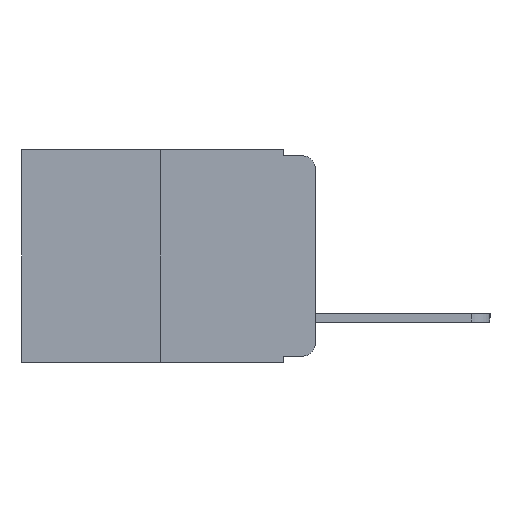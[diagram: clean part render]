
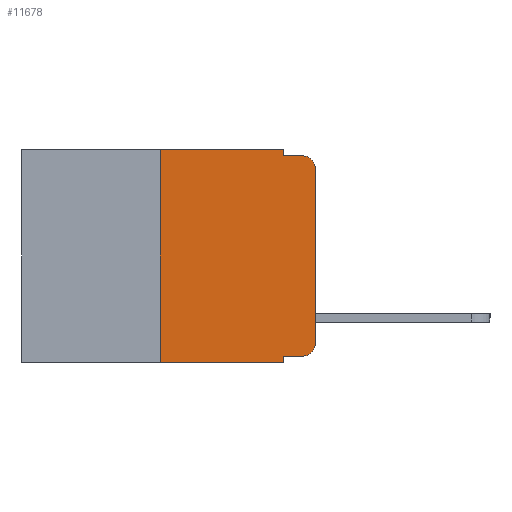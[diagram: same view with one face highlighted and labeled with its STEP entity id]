
A CAD part, left-side view. The second image highlights one B-rep face of the part: STEP entity #11678.
In plain terms, the highlighted planar face has unit normal (-1, 0, 0).
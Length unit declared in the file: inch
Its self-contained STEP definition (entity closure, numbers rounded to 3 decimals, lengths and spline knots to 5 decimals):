
#26 = DIRECTION ( 'NONE',  ( 0., 0., -1. ) ) ;
#235 = ORIENTED_EDGE ( 'NONE', *, *, #14820, .F. ) ;
#338 = DIRECTION ( 'NONE',  ( 1., 0., 0. ) ) ;
#507 = CARTESIAN_POINT ( 'NONE',  ( 0., 0.02, -0.01 ) ) ;
#1001 = DIRECTION ( 'NONE',  ( 0., -1., 0. ) ) ;
#1070 = ORIENTED_EDGE ( 'NONE', *, *, #17965, .F. ) ;
#1415 = DIRECTION ( 'NONE',  ( 0., 0., -1. ) ) ;
#1560 = CARTESIAN_POINT ( 'NONE',  ( 0., 0., 0. ) ) ;
#1815 = CARTESIAN_POINT ( 'NONE',  ( 0., 0.25, -0.343 ) ) ;
#1940 = VERTEX_POINT ( 'NONE', #16878 ) ;
#2002 = PLANE ( 'NONE',  #14987 ) ;
#2041 = VECTOR ( 'NONE', #6393, 39.37008 ) ;
#2504 = EDGE_CURVE ( 'NONE', #9004, #8777, #14650, .T. ) ;
#2697 = VERTEX_POINT ( 'NONE', #507 ) ;
#2746 = CARTESIAN_POINT ( 'NONE',  ( 0., 0.051, -0.333 ) ) ;
#2930 = ORIENTED_EDGE ( 'NONE', *, *, #12748, .T. ) ;
#2942 = FACE_OUTER_BOUND ( 'NONE', #18625, .T. ) ;
#4654 = VERTEX_POINT ( 'NONE', #9263 ) ;
#5141 = DIRECTION ( 'NONE',  ( 0., 0., 1. ) ) ;
#5259 = CARTESIAN_POINT ( 'NONE',  ( 0., 0.051, -0.01 ) ) ;
#5276 = VERTEX_POINT ( 'NONE', #15766 ) ;
#5725 = ORIENTED_EDGE ( 'NONE', *, *, #13641, .T. ) ;
#5962 = LINE ( 'NONE', #2746, #14528 ) ;
#5964 = LINE ( 'NONE', #11373, #14036 ) ;
#6369 = VECTOR ( 'NONE', #18024, 39.37008 ) ;
#6393 = DIRECTION ( 'NONE',  ( 0., 0., -1. ) ) ;
#6933 = CARTESIAN_POINT ( 'NONE',  ( 0., 0.473, 0. ) ) ;
#6975 = DIRECTION ( 'NONE',  ( 0., -1., 0. ) ) ;
#7936 = DIRECTION ( 'NONE',  ( 0., 0., -1. ) ) ;
#8777 = VERTEX_POINT ( 'NONE', #18699 ) ;
#8801 = CARTESIAN_POINT ( 'NONE',  ( 0., 0.051, -0.343 ) ) ;
#8851 = LINE ( 'NONE', #9237, #20805 ) ;
#9004 = VERTEX_POINT ( 'NONE', #17749 ) ;
#9237 = CARTESIAN_POINT ( 'NONE',  ( 0., 0.473, -0.343 ) ) ;
#9263 = CARTESIAN_POINT ( 'NONE',  ( 0., 0.051, -0.01 ) ) ;
#9523 = EDGE_CURVE ( 'NONE', #19681, #9004, #12698, .T. ) ;
#9581 = CARTESIAN_POINT ( 'NONE',  ( 0., 0.051, 0. ) ) ;
#9985 = DIRECTION ( 'NONE',  ( -1., 0., 0. ) ) ;
#10102 = VECTOR ( 'NONE', #7936, 39.37008 ) ;
#10228 = LINE ( 'NONE', #5259, #6369 ) ;
#10261 = LINE ( 'NONE', #14430, #2041 ) ;
#10433 = VECTOR ( 'NONE', #5141, 39.37008 ) ;
#10814 = CARTESIAN_POINT ( 'NONE',  ( 0., 0.051, 0. ) ) ;
#11120 = AXIS2_PLACEMENT_3D ( 'NONE', #20524, #11228, #1415 ) ;
#11228 = DIRECTION ( 'NONE',  ( -1., 0., 0. ) ) ;
#11373 = CARTESIAN_POINT ( 'NONE',  ( 0., 0.25, 0. ) ) ;
#11595 = ORIENTED_EDGE ( 'NONE', *, *, #9523, .T. ) ;
#11678 = ADVANCED_FACE ( 'NONE', ( #2942 ), #2002, .F. ) ;
#11856 = DIRECTION ( 'NONE',  ( 0., 0., -1. ) ) ;
#12392 = VECTOR ( 'NONE', #6975, 39.37008 ) ;
#12394 = VERTEX_POINT ( 'NONE', #1815 ) ;
#12698 = CIRCLE ( 'NONE', #11120, 0.02 ) ;
#12748 = EDGE_CURVE ( 'NONE', #5276, #19681, #5962, .T. ) ;
#12841 = ORIENTED_EDGE ( 'NONE', *, *, #13441, .F. ) ;
#12970 = DIRECTION ( 'NONE',  ( 0., 0., 1. ) ) ;
#13441 = EDGE_CURVE ( 'NONE', #1940, #14596, #16560, .T. ) ;
#13491 = VERTEX_POINT ( 'NONE', #8801 ) ;
#13641 = EDGE_CURVE ( 'NONE', #12394, #13491, #8851, .T. ) ;
#13760 = EDGE_CURVE ( 'NONE', #5276, #13491, #15315, .T. ) ;
#14011 = AXIS2_PLACEMENT_3D ( 'NONE', #19357, #9985, #26 ) ;
#14036 = VECTOR ( 'NONE', #12970, 39.37008 ) ;
#14062 = DIRECTION ( 'NONE',  ( 0., -1., 0. ) ) ;
#14430 = CARTESIAN_POINT ( 'NONE',  ( 0., 0.051, 0. ) ) ;
#14514 = ORIENTED_EDGE ( 'NONE', *, *, #2504, .T. ) ;
#14528 = VECTOR ( 'NONE', #14062, 39.37008 ) ;
#14534 = ORIENTED_EDGE ( 'NONE', *, *, #16960, .F. ) ;
#14596 = VERTEX_POINT ( 'NONE', #10814 ) ;
#14650 = LINE ( 'NONE', #1560, #10433 ) ;
#14820 = EDGE_CURVE ( 'NONE', #12394, #1940, #5964, .T. ) ;
#14862 = CIRCLE ( 'NONE', #14011, 0.02 ) ;
#14987 = AXIS2_PLACEMENT_3D ( 'NONE', #6933, #338, #11856 ) ;
#15315 = LINE ( 'NONE', #9581, #10102 ) ;
#15766 = CARTESIAN_POINT ( 'NONE',  ( 0., 0.051, -0.333 ) ) ;
#16017 = ORIENTED_EDGE ( 'NONE', *, *, #19982, .T. ) ;
#16560 = LINE ( 'NONE', #18120, #12392 ) ;
#16878 = CARTESIAN_POINT ( 'NONE',  ( 0., 0.25, 0. ) ) ;
#16960 = EDGE_CURVE ( 'NONE', #14596, #4654, #10261, .T. ) ;
#17749 = CARTESIAN_POINT ( 'NONE',  ( 0., 0., -0.313 ) ) ;
#17965 = EDGE_CURVE ( 'NONE', #4654, #2697, #10228, .T. ) ;
#18024 = DIRECTION ( 'NONE',  ( 0., -1., 0. ) ) ;
#18120 = CARTESIAN_POINT ( 'NONE',  ( 0., 0.473, 0. ) ) ;
#18625 = EDGE_LOOP ( 'NONE', ( #14514, #16017, #1070, #14534, #12841, #235, #5725, #18938, #2930, #11595 ) ) ;
#18699 = CARTESIAN_POINT ( 'NONE',  ( 0., 0., -0.03 ) ) ;
#18938 = ORIENTED_EDGE ( 'NONE', *, *, #13760, .F. ) ;
#19357 = CARTESIAN_POINT ( 'NONE',  ( 0., 0.02, -0.03 ) ) ;
#19681 = VERTEX_POINT ( 'NONE', #20152 ) ;
#19982 = EDGE_CURVE ( 'NONE', #8777, #2697, #14862, .T. ) ;
#20152 = CARTESIAN_POINT ( 'NONE',  ( 0., 0.02, -0.333 ) ) ;
#20524 = CARTESIAN_POINT ( 'NONE',  ( 0., 0.02, -0.313 ) ) ;
#20805 = VECTOR ( 'NONE', #1001, 39.37008 ) ;
